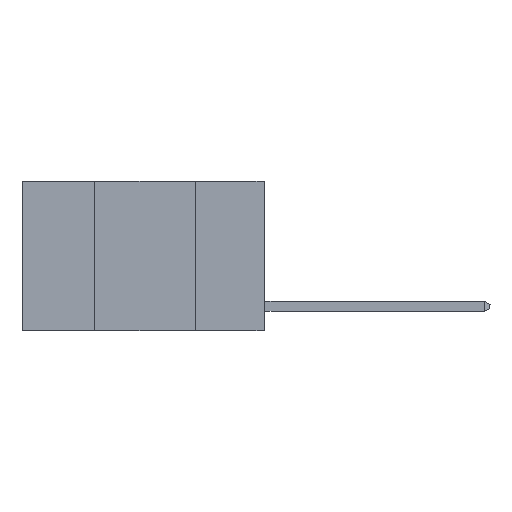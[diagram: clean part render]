
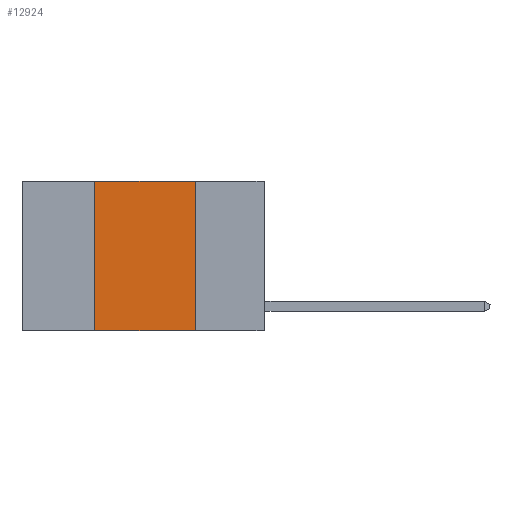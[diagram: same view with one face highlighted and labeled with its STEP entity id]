
A CAD part, left-side view. The second image highlights one B-rep face of the part: STEP entity #12924.
In plain terms, the highlighted planar face has unit normal (-1, 0, 0).
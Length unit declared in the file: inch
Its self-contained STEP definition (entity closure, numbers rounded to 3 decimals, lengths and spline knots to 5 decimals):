
#142 = DIRECTION ( 'NONE',  ( 0., 0., 1. ) ) ;
#1042 = VECTOR ( 'NONE', #6715, 39.37008 ) ;
#1692 = ORIENTED_EDGE ( 'NONE', *, *, #3522, .F. ) ;
#1831 = VERTEX_POINT ( 'NONE', #4433 ) ;
#3122 = CARTESIAN_POINT ( 'NONE',  ( 0., 0.17, 0. ) ) ;
#3522 = EDGE_CURVE ( 'NONE', #16589, #1831, #11774, .T. ) ;
#3623 = VECTOR ( 'NONE', #9818, 39.37008 ) ;
#3652 = EDGE_CURVE ( 'NONE', #11465, #4605, #9726, .T. ) ;
#3848 = LINE ( 'NONE', #9661, #1042 ) ;
#4377 = ORIENTED_EDGE ( 'NONE', *, *, #3652, .F. ) ;
#4433 = CARTESIAN_POINT ( 'NONE',  ( 0., 0.42, 0. ) ) ;
#4605 = VERTEX_POINT ( 'NONE', #18379 ) ;
#4631 = CARTESIAN_POINT ( 'NONE',  ( 0., 0.42, 0. ) ) ;
#4836 = VECTOR ( 'NONE', #142, 39.37008 ) ;
#5249 = CARTESIAN_POINT ( 'NONE',  ( 0., 0.17, 0. ) ) ;
#5434 = DIRECTION ( 'NONE',  ( 0., 0., -1. ) ) ;
#5454 = ORIENTED_EDGE ( 'NONE', *, *, #17276, .T. ) ;
#6171 = EDGE_CURVE ( 'NONE', #1831, #11465, #3848, .T. ) ;
#6715 = DIRECTION ( 'NONE',  ( 0., -1., 0. ) ) ;
#6864 = FACE_OUTER_BOUND ( 'NONE', #14542, .T. ) ;
#9661 = CARTESIAN_POINT ( 'NONE',  ( 0., 0.6, 0. ) ) ;
#9726 = LINE ( 'NONE', #5249, #3623 ) ;
#9808 = DIRECTION ( 'NONE',  ( 1., 0., 0. ) ) ;
#9818 = DIRECTION ( 'NONE',  ( 0., 0., -1. ) ) ;
#11465 = VERTEX_POINT ( 'NONE', #3122 ) ;
#11479 = CARTESIAN_POINT ( 'NONE',  ( 0., 0.6, -0.37 ) ) ;
#11774 = LINE ( 'NONE', #4631, #4836 ) ;
#12680 = PLANE ( 'NONE',  #17091 ) ;
#12924 = ADVANCED_FACE ( 'NONE', ( #6864 ), #12680, .F. ) ;
#14008 = ORIENTED_EDGE ( 'NONE', *, *, #6171, .F. ) ;
#14542 = EDGE_LOOP ( 'NONE', ( #4377, #14008, #1692, #5454 ) ) ;
#16049 = CARTESIAN_POINT ( 'NONE',  ( 0., 0.42, -0.37 ) ) ;
#16589 = VERTEX_POINT ( 'NONE', #16049 ) ;
#17091 = AXIS2_PLACEMENT_3D ( 'NONE', #18510, #9808, #5434 ) ;
#17276 = EDGE_CURVE ( 'NONE', #16589, #4605, #18557, .T. ) ;
#17326 = DIRECTION ( 'NONE',  ( 0., -1., 0. ) ) ;
#17474 = VECTOR ( 'NONE', #17326, 39.37008 ) ;
#18379 = CARTESIAN_POINT ( 'NONE',  ( 0., 0.17, -0.37 ) ) ;
#18510 = CARTESIAN_POINT ( 'NONE',  ( 0., 0.6, 0. ) ) ;
#18557 = LINE ( 'NONE', #11479, #17474 ) ;
